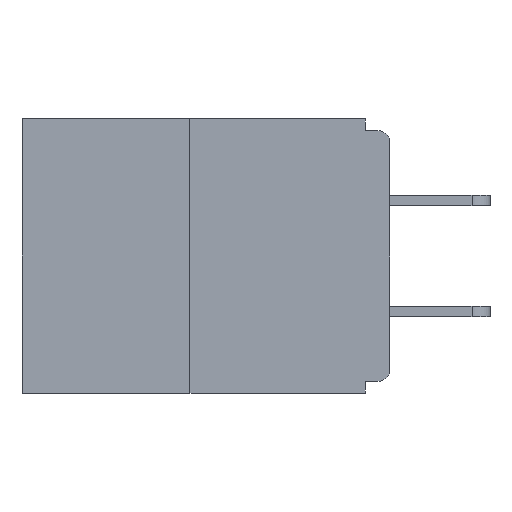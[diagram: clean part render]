
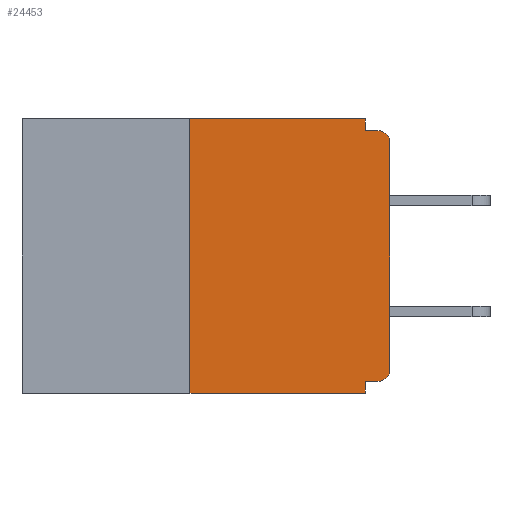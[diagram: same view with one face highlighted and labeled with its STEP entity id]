
A CAD part, left-side view. The second image highlights one B-rep face of the part: STEP entity #24453.
In plain terms, the highlighted planar face has unit normal (-1, 0, 0).
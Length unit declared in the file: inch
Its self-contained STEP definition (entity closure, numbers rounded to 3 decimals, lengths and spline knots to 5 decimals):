
#450 = CARTESIAN_POINT ( 'NONE',  ( 0., 0.015, -0.328 ) ) ;
#551 = VERTEX_POINT ( 'NONE', #14392 ) ;
#736 = ORIENTED_EDGE ( 'NONE', *, *, #18468, .F. ) ;
#1466 = AXIS2_PLACEMENT_3D ( 'NONE', #8505, #19158, #23314 ) ;
#1710 = LINE ( 'NONE', #21515, #9323 ) ;
#3425 = LINE ( 'NONE', #4132, #4394 ) ;
#3580 = ORIENTED_EDGE ( 'NONE', *, *, #17144, .F. ) ;
#3876 = CARTESIAN_POINT ( 'NONE',  ( 0., 0.031, 0. ) ) ;
#3883 = EDGE_CURVE ( 'NONE', #24543, #27465, #11925, .T. ) ;
#4093 = DIRECTION ( 'NONE',  ( 0., 0., -1. ) ) ;
#4124 = ORIENTED_EDGE ( 'NONE', *, *, #3883, .T. ) ;
#4132 = CARTESIAN_POINT ( 'NONE',  ( 0., 0.031, -0.343 ) ) ;
#4233 = PLANE ( 'NONE',  #1466 ) ;
#4265 = LINE ( 'NONE', #5235, #4932 ) ;
#4394 = VECTOR ( 'NONE', #10608, 39.37008 ) ;
#4555 = VERTEX_POINT ( 'NONE', #21133 ) ;
#4760 = DIRECTION ( 'NONE',  ( 0., -1., 0. ) ) ;
#4865 = CARTESIAN_POINT ( 'NONE',  ( 0., 0., -0.313 ) ) ;
#4932 = VECTOR ( 'NONE', #20039, 39.37008 ) ;
#5079 = VECTOR ( 'NONE', #19416, 39.37008 ) ;
#5235 = CARTESIAN_POINT ( 'NONE',  ( 0., 0.031, 0. ) ) ;
#5722 = ORIENTED_EDGE ( 'NONE', *, *, #7531, .F. ) ;
#5727 = VECTOR ( 'NONE', #25859, 39.37008 ) ;
#6763 = EDGE_CURVE ( 'NONE', #27465, #4555, #21407, .T. ) ;
#7133 = ORIENTED_EDGE ( 'NONE', *, *, #26693, .T. ) ;
#7531 = EDGE_CURVE ( 'NONE', #24543, #551, #11760, .T. ) ;
#7563 = DIRECTION ( 'NONE',  ( 0., 0., 1. ) ) ;
#8152 = ORIENTED_EDGE ( 'NONE', *, *, #18864, .F. ) ;
#8458 = ORIENTED_EDGE ( 'NONE', *, *, #23576, .T. ) ;
#8505 = CARTESIAN_POINT ( 'NONE',  ( 0., 0.46, 0. ) ) ;
#9073 = CARTESIAN_POINT ( 'NONE',  ( 0., 0.015, -0.313 ) ) ;
#9323 = VECTOR ( 'NONE', #4760, 39.37008 ) ;
#9395 = VERTEX_POINT ( 'NONE', #16276 ) ;
#9450 = ORIENTED_EDGE ( 'NONE', *, *, #24637, .F. ) ;
#9633 = ORIENTED_EDGE ( 'NONE', *, *, #6763, .T. ) ;
#10608 = DIRECTION ( 'NONE',  ( 0., 0., -1. ) ) ;
#10616 = DIRECTION ( 'NONE',  ( 0., 1., 0. ) ) ;
#10720 = LINE ( 'NONE', #23668, #5079 ) ;
#11207 = DIRECTION ( 'NONE',  ( 0., 0., -1. ) ) ;
#11760 = LINE ( 'NONE', #19145, #20722 ) ;
#11925 = CIRCLE ( 'NONE', #15740, 0.015 ) ;
#12442 = VERTEX_POINT ( 'NONE', #22424 ) ;
#12574 = ORIENTED_EDGE ( 'NONE', *, *, #19468, .F. ) ;
#12928 = VERTEX_POINT ( 'NONE', #22487 ) ;
#13076 = LINE ( 'NONE', #13091, #23388 ) ;
#13091 = CARTESIAN_POINT ( 'NONE',  ( 0., 0.46, 0. ) ) ;
#13647 = LINE ( 'NONE', #21561, #5727 ) ;
#14007 = VERTEX_POINT ( 'NONE', #3876 ) ;
#14242 = EDGE_LOOP ( 'NONE', ( #3580, #8152, #8458, #12574, #5722, #4124, #9633, #7133, #736, #9450 ) ) ;
#14382 = CIRCLE ( 'NONE', #24924, 0.015 ) ;
#14392 = CARTESIAN_POINT ( 'NONE',  ( 0., 0.031, -0.328 ) ) ;
#14633 = DIRECTION ( 'NONE',  ( -1., 0., 0. ) ) ;
#15740 = AXIS2_PLACEMENT_3D ( 'NONE', #9073, #23885, #11207 ) ;
#16262 = CARTESIAN_POINT ( 'NONE',  ( 0., 0., 0. ) ) ;
#16276 = CARTESIAN_POINT ( 'NONE',  ( 0., 0.015, -0.015 ) ) ;
#17144 = EDGE_CURVE ( 'NONE', #23893, #14007, #13076, .T. ) ;
#17465 = CARTESIAN_POINT ( 'NONE',  ( 0., 0.25, -0.343 ) ) ;
#18468 = EDGE_CURVE ( 'NONE', #12928, #9395, #10720, .T. ) ;
#18864 = EDGE_CURVE ( 'NONE', #25783, #23893, #13647, .T. ) ;
#19145 = CARTESIAN_POINT ( 'NONE',  ( 0., 0., -0.328 ) ) ;
#19158 = DIRECTION ( 'NONE',  ( 1., 0., 0. ) ) ;
#19416 = DIRECTION ( 'NONE',  ( 0., -1., 0. ) ) ;
#19468 = EDGE_CURVE ( 'NONE', #551, #12442, #3425, .T. ) ;
#20039 = DIRECTION ( 'NONE',  ( 0., 0., -1. ) ) ;
#20169 = FACE_OUTER_BOUND ( 'NONE', #14242, .T. ) ;
#20722 = VECTOR ( 'NONE', #10616, 39.37008 ) ;
#21133 = CARTESIAN_POINT ( 'NONE',  ( 0., 0., -0.03 ) ) ;
#21407 = LINE ( 'NONE', #16262, #26107 ) ;
#21515 = CARTESIAN_POINT ( 'NONE',  ( 0., 0.46, -0.343 ) ) ;
#21561 = CARTESIAN_POINT ( 'NONE',  ( 0., 0.25, 0. ) ) ;
#22424 = CARTESIAN_POINT ( 'NONE',  ( 0., 0.031, -0.343 ) ) ;
#22487 = CARTESIAN_POINT ( 'NONE',  ( 0., 0.031, -0.015 ) ) ;
#23314 = DIRECTION ( 'NONE',  ( 0., 0., -1. ) ) ;
#23388 = VECTOR ( 'NONE', #25659, 39.37008 ) ;
#23576 = EDGE_CURVE ( 'NONE', #25783, #12442, #1710, .T. ) ;
#23668 = CARTESIAN_POINT ( 'NONE',  ( 0., 0., -0.015 ) ) ;
#23885 = DIRECTION ( 'NONE',  ( -1., 0., 0. ) ) ;
#23893 = VERTEX_POINT ( 'NONE', #25982 ) ;
#24453 = ADVANCED_FACE ( 'NONE', ( #20169 ), #4233, .F. ) ;
#24543 = VERTEX_POINT ( 'NONE', #450 ) ;
#24637 = EDGE_CURVE ( 'NONE', #14007, #12928, #4265, .T. ) ;
#24924 = AXIS2_PLACEMENT_3D ( 'NONE', #27405, #14633, #4093 ) ;
#25659 = DIRECTION ( 'NONE',  ( 0., -1., 0. ) ) ;
#25783 = VERTEX_POINT ( 'NONE', #17465 ) ;
#25859 = DIRECTION ( 'NONE',  ( 0., 0., 1. ) ) ;
#25982 = CARTESIAN_POINT ( 'NONE',  ( 0., 0.25, 0. ) ) ;
#26107 = VECTOR ( 'NONE', #7563, 39.37008 ) ;
#26693 = EDGE_CURVE ( 'NONE', #4555, #9395, #14382, .T. ) ;
#27405 = CARTESIAN_POINT ( 'NONE',  ( 0., 0.015, -0.03 ) ) ;
#27465 = VERTEX_POINT ( 'NONE', #4865 ) ;
